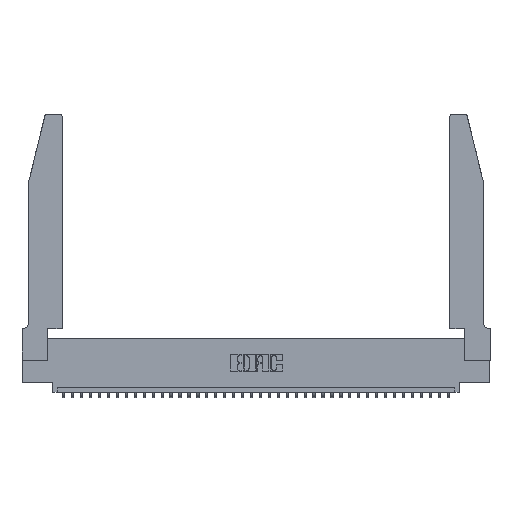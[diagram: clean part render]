
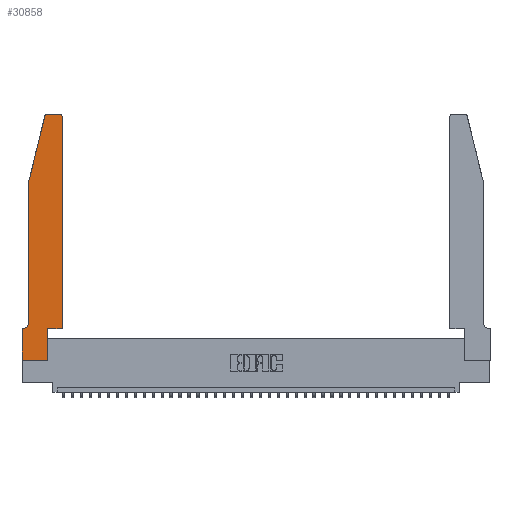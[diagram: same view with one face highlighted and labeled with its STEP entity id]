
A CAD part, top view. The second image highlights one B-rep face of the part: STEP entity #30858.
In plain terms, the highlighted planar face has unit normal (0, 0, 1).
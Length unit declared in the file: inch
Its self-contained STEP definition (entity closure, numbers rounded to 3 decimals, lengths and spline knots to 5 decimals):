
#182 = EDGE_CURVE ( 'NONE', #36790, #34425, #22858, .T. ) ;
#330 = VECTOR ( 'NONE', #3470, 39.37008 ) ;
#1188 = DIRECTION ( 'NONE',  ( -1., 0., 0. ) ) ;
#2145 = CARTESIAN_POINT ( 'NONE',  ( 0.2865, 0.35, 0.37 ) ) ;
#2180 = DIRECTION ( 'NONE',  ( -0.239, -0.971, 0. ) ) ;
#2280 = CARTESIAN_POINT ( 'NONE',  ( 0., 0.35, 0.37 ) ) ;
#2300 = CARTESIAN_POINT ( 'NONE',  ( 0.4205, 2.75, 0.37 ) ) ;
#2414 = EDGE_CURVE ( 'NONE', #35313, #36790, #8542, .T. ) ;
#2563 = EDGE_CURVE ( 'NONE', #31520, #35313, #29512, .T. ) ;
#2899 = DIRECTION ( 'NONE',  ( 0., 0., 1. ) ) ;
#3325 = CARTESIAN_POINT ( 'NONE',  ( 0.4505, 0.35, 0.37 ) ) ;
#3470 = DIRECTION ( 'NONE',  ( -1., 0., 0. ) ) ;
#3773 = EDGE_CURVE ( 'NONE', #36374, #31160, #6562, .T. ) ;
#4095 = VECTOR ( 'NONE', #35787, 39.37008 ) ;
#4576 = EDGE_CURVE ( 'NONE', #25799, #31520, #5629, .T. ) ;
#4898 = DIRECTION ( 'NONE',  ( 0., 0., 1. ) ) ;
#5077 = CARTESIAN_POINT ( 'NONE',  ( 0.0755, 2., 0.37 ) ) ;
#5629 = CIRCLE ( 'NONE', #25953, 0.03 ) ;
#5727 = EDGE_CURVE ( 'NONE', #26957, #36374, #36699, .T. ) ;
#6054 = CARTESIAN_POINT ( 'NONE',  ( 0., 0., 0.37 ) ) ;
#6562 = CIRCLE ( 'NONE', #26904, 0.03 ) ;
#6815 = CARTESIAN_POINT ( 'NONE',  ( 0.25487, 2.72718, 0.37 ) ) ;
#7546 = DIRECTION ( 'NONE',  ( 0., 0., -1. ) ) ;
#8191 = VECTOR ( 'NONE', #21822, 39.37008 ) ;
#8542 = LINE ( 'NONE', #20620, #17629 ) ;
#9326 = CARTESIAN_POINT ( 'NONE',  ( 0.2865, 0.35, 0.37 ) ) ;
#9874 = EDGE_LOOP ( 'NONE', ( #28484, #18473, #14918, #17208, #22900, #24019, #22786, #25612, #37314, #10590, #11665, #23040 ) ) ;
#9880 = EDGE_CURVE ( 'NONE', #31211, #24975, #29505, .T. ) ;
#10590 = ORIENTED_EDGE ( 'NONE', *, *, #18156, .T. ) ;
#10633 = PLANE ( 'NONE',  #34131 ) ;
#11098 = DIRECTION ( 'NONE',  ( 0., 1., 0. ) ) ;
#11151 = CARTESIAN_POINT ( 'NONE',  ( 0.4205, 2.72, 0.37 ) ) ;
#11570 = EDGE_CURVE ( 'NONE', #35297, #31191, #19340, .T. ) ;
#11665 = ORIENTED_EDGE ( 'NONE', *, *, #5727, .T. ) ;
#11994 = CARTESIAN_POINT ( 'NONE',  ( 0.4505, 0.35, 0.37 ) ) ;
#12101 = VECTOR ( 'NONE', #11098, 39.37008 ) ;
#12617 = LINE ( 'NONE', #24816, #330 ) ;
#12760 = CARTESIAN_POINT ( 'NONE',  ( 0.0055, 0.42, 0.37 ) ) ;
#13843 = DIRECTION ( 'NONE',  ( 0., 0., 1. ) ) ;
#13985 = CARTESIAN_POINT ( 'NONE',  ( 0.4505, 2.72, 0.37 ) ) ;
#14918 = ORIENTED_EDGE ( 'NONE', *, *, #2563, .T. ) ;
#16822 = CARTESIAN_POINT ( 'NONE',  ( 0., 0., 0.37 ) ) ;
#17071 = FACE_OUTER_BOUND ( 'NONE', #9874, .T. ) ;
#17208 = ORIENTED_EDGE ( 'NONE', *, *, #2414, .T. ) ;
#17258 = EDGE_CURVE ( 'NONE', #31191, #31211, #21399, .T. ) ;
#17629 = VECTOR ( 'NONE', #29228, 39.37008 ) ;
#17633 = DIRECTION ( 'NONE',  ( 0., 1., 0. ) ) ;
#18156 = EDGE_CURVE ( 'NONE', #24975, #26957, #21318, .T. ) ;
#18473 = ORIENTED_EDGE ( 'NONE', *, *, #4576, .T. ) ;
#18520 = AXIS2_PLACEMENT_3D ( 'NONE', #12760, #7546, #1188 ) ;
#19340 = LINE ( 'NONE', #6054, #28500 ) ;
#19456 = DIRECTION ( 'NONE',  ( 1., 0., 0. ) ) ;
#20465 = CARTESIAN_POINT ( 'NONE',  ( 0.2865, 0., 0.37 ) ) ;
#20620 = CARTESIAN_POINT ( 'NONE',  ( 0.0755, 2., 0.37 ) ) ;
#21171 = CARTESIAN_POINT ( 'NONE',  ( 0., 0., 0.37 ) ) ;
#21288 = CARTESIAN_POINT ( 'NONE',  ( 0.0755, 0.35, 0.37 ) ) ;
#21318 = LINE ( 'NONE', #3325, #36940 ) ;
#21399 = LINE ( 'NONE', #21171, #4095 ) ;
#21822 = DIRECTION ( 'NONE',  ( -1., 0., 0. ) ) ;
#22104 = DIRECTION ( 'NONE',  ( 1., 0., 0. ) ) ;
#22140 = CARTESIAN_POINT ( 'NONE',  ( 0.0755, 0.42, 0.37 ) ) ;
#22786 = ORIENTED_EDGE ( 'NONE', *, *, #11570, .T. ) ;
#22858 = CIRCLE ( 'NONE', #18520, 0.07 ) ;
#22900 = ORIENTED_EDGE ( 'NONE', *, *, #182, .T. ) ;
#23040 = ORIENTED_EDGE ( 'NONE', *, *, #3773, .T. ) ;
#23733 = EDGE_CURVE ( 'NONE', #31160, #25799, #12617, .T. ) ;
#23764 = DIRECTION ( 'NONE',  ( 1., 0., 0. ) ) ;
#24019 = ORIENTED_EDGE ( 'NONE', *, *, #27739, .T. ) ;
#24033 = DIRECTION ( 'NONE',  ( 0., -1., 0. ) ) ;
#24816 = CARTESIAN_POINT ( 'NONE',  ( 0.2605, 2.75, 0.37 ) ) ;
#24975 = VERTEX_POINT ( 'NONE', #9326 ) ;
#25612 = ORIENTED_EDGE ( 'NONE', *, *, #17258, .T. ) ;
#25799 = VERTEX_POINT ( 'NONE', #35445 ) ;
#25953 = AXIS2_PLACEMENT_3D ( 'NONE', #34320, #2899, #23764 ) ;
#26904 = AXIS2_PLACEMENT_3D ( 'NONE', #11151, #13843, #19456 ) ;
#26957 = VERTEX_POINT ( 'NONE', #36189 ) ;
#27413 = LINE ( 'NONE', #21288, #8191 ) ;
#27739 = EDGE_CURVE ( 'NONE', #34425, #35297, #27413, .T. ) ;
#28484 = ORIENTED_EDGE ( 'NONE', *, *, #23733, .T. ) ;
#28500 = VECTOR ( 'NONE', #24033, 39.37008 ) ;
#28902 = VECTOR ( 'NONE', #17633, 39.37008 ) ;
#29228 = DIRECTION ( 'NONE',  ( 0., -1., 0. ) ) ;
#29505 = LINE ( 'NONE', #2145, #12101 ) ;
#29512 = LINE ( 'NONE', #31680, #36864 ) ;
#30858 = ADVANCED_FACE ( 'NONE', ( #17071 ), #10633, .T. ) ;
#31160 = VERTEX_POINT ( 'NONE', #2300 ) ;
#31191 = VERTEX_POINT ( 'NONE', #16822 ) ;
#31211 = VERTEX_POINT ( 'NONE', #20465 ) ;
#31520 = VERTEX_POINT ( 'NONE', #6815 ) ;
#31680 = CARTESIAN_POINT ( 'NONE',  ( 0.0755, 2., 0.37 ) ) ;
#32706 = DIRECTION ( 'NONE',  ( 1., 0., 0. ) ) ;
#33637 = CARTESIAN_POINT ( 'NONE',  ( 0., 0.35, 0.37 ) ) ;
#34131 = AXIS2_PLACEMENT_3D ( 'NONE', #33637, #4898, #22104 ) ;
#34320 = CARTESIAN_POINT ( 'NONE',  ( 0.284, 2.72, 0.37 ) ) ;
#34425 = VERTEX_POINT ( 'NONE', #36164 ) ;
#35297 = VERTEX_POINT ( 'NONE', #2280 ) ;
#35313 = VERTEX_POINT ( 'NONE', #5077 ) ;
#35445 = CARTESIAN_POINT ( 'NONE',  ( 0.284, 2.75, 0.37 ) ) ;
#35787 = DIRECTION ( 'NONE',  ( 1., 0., 0. ) ) ;
#36164 = CARTESIAN_POINT ( 'NONE',  ( 0.0055, 0.35, 0.37 ) ) ;
#36189 = CARTESIAN_POINT ( 'NONE',  ( 0.4505, 0.35, 0.37 ) ) ;
#36374 = VERTEX_POINT ( 'NONE', #13985 ) ;
#36699 = LINE ( 'NONE', #11994, #28902 ) ;
#36790 = VERTEX_POINT ( 'NONE', #22140 ) ;
#36864 = VECTOR ( 'NONE', #2180, 39.37008 ) ;
#36940 = VECTOR ( 'NONE', #32706, 39.37008 ) ;
#37314 = ORIENTED_EDGE ( 'NONE', *, *, #9880, .T. ) ;
